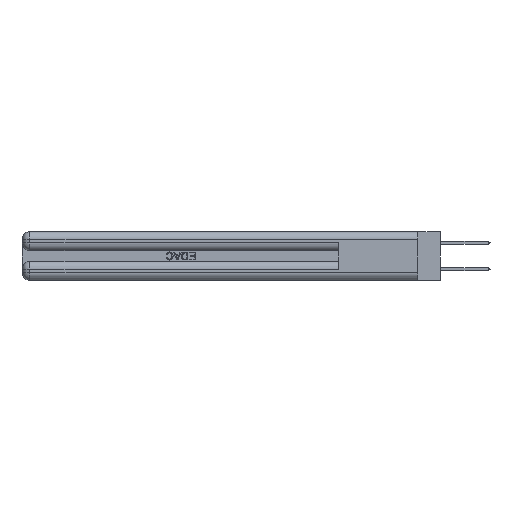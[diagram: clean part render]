
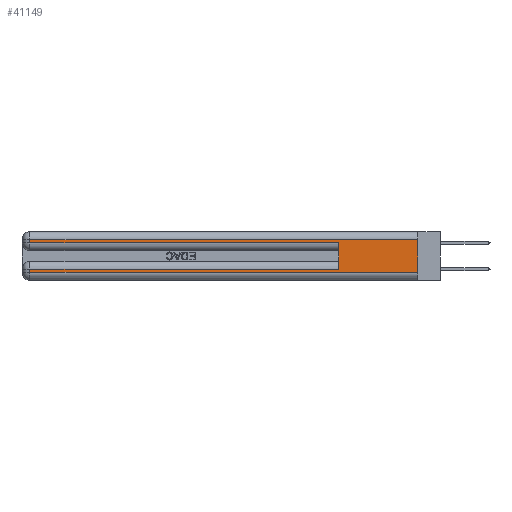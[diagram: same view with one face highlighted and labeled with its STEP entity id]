
A CAD part, left-side view. The second image highlights one B-rep face of the part: STEP entity #41149.
In plain terms, the highlighted planar face has unit normal (-1, 0, 0).
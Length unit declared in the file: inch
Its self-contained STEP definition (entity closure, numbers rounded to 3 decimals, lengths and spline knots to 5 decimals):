
#847 = CARTESIAN_POINT ( 'NONE',  ( 0., 0.6, 0.285 ) ) ;
#1053 = ORIENTED_EDGE ( 'NONE', *, *, #19100, .T. ) ;
#1753 = CARTESIAN_POINT ( 'NONE',  ( 0., 0., 0.06 ) ) ;
#2328 = LINE ( 'NONE', #5971, #9478 ) ;
#3361 = VERTEX_POINT ( 'NONE', #847 ) ;
#4598 = CARTESIAN_POINT ( 'NONE',  ( 0., 0., 0.37 ) ) ;
#5028 = VERTEX_POINT ( 'NONE', #23712 ) ;
#5296 = CARTESIAN_POINT ( 'NONE',  ( 0., 0., 0.37 ) ) ;
#5336 = EDGE_CURVE ( 'NONE', #12932, #10957, #39170, .T. ) ;
#5971 = CARTESIAN_POINT ( 'NONE',  ( 0., 0., 0.06 ) ) ;
#6801 = EDGE_CURVE ( 'NONE', #10957, #3361, #25562, .T. ) ;
#6872 = CARTESIAN_POINT ( 'NONE',  ( 0., 2.94, 0.085 ) ) ;
#7126 = ORIENTED_EDGE ( 'NONE', *, *, #5336, .T. ) ;
#7146 = VECTOR ( 'NONE', #8077, 39.37008 ) ;
#8077 = DIRECTION ( 'NONE',  ( 0., -1., 0. ) ) ;
#8470 = CARTESIAN_POINT ( 'NONE',  ( 0., 2.94, 0.285 ) ) ;
#9478 = VECTOR ( 'NONE', #9497, 39.37008 ) ;
#9497 = DIRECTION ( 'NONE',  ( 0., -1., 0. ) ) ;
#9803 = CARTESIAN_POINT ( 'NONE',  ( 0., 0., 0.085 ) ) ;
#10957 = VERTEX_POINT ( 'NONE', #8470 ) ;
#11416 = CARTESIAN_POINT ( 'NONE',  ( 0., 0., 0.285 ) ) ;
#11647 = VECTOR ( 'NONE', #25350, 39.37008 ) ;
#11980 = VERTEX_POINT ( 'NONE', #13518 ) ;
#12282 = VECTOR ( 'NONE', #25391, 39.37008 ) ;
#12932 = VERTEX_POINT ( 'NONE', #16502 ) ;
#13084 = ORIENTED_EDGE ( 'NONE', *, *, #43287, .F. ) ;
#13295 = DIRECTION ( 'NONE',  ( 0., 1., 0. ) ) ;
#13518 = CARTESIAN_POINT ( 'NONE',  ( 0., 2.94, 0.06 ) ) ;
#15785 = DIRECTION ( 'NONE',  ( 0., 0., -1. ) ) ;
#16337 = ORIENTED_EDGE ( 'NONE', *, *, #6801, .T. ) ;
#16502 = CARTESIAN_POINT ( 'NONE',  ( 0., 2.94, 0.31 ) ) ;
#16762 = EDGE_CURVE ( 'NONE', #18820, #33430, #39166, .T. ) ;
#17178 = DIRECTION ( 'NONE',  ( 0., 0., 1. ) ) ;
#17978 = ORIENTED_EDGE ( 'NONE', *, *, #25592, .F. ) ;
#18076 = LINE ( 'NONE', #38897, #44460 ) ;
#18519 = ORIENTED_EDGE ( 'NONE', *, *, #16762, .T. ) ;
#18820 = VERTEX_POINT ( 'NONE', #43369 ) ;
#19100 = EDGE_CURVE ( 'NONE', #33430, #11980, #21241, .T. ) ;
#19742 = VECTOR ( 'NONE', #13295, 39.37008 ) ;
#20513 = CARTESIAN_POINT ( 'NONE',  ( 0., 0.6, 0.145 ) ) ;
#21241 = LINE ( 'NONE', #41396, #38496 ) ;
#23015 = EDGE_CURVE ( 'NONE', #11980, #39337, #2328, .T. ) ;
#23712 = CARTESIAN_POINT ( 'NONE',  ( 0., 0., 0.31 ) ) ;
#24948 = VECTOR ( 'NONE', #17178, 39.37008 ) ;
#25350 = DIRECTION ( 'NONE',  ( 0., 0., -1. ) ) ;
#25391 = DIRECTION ( 'NONE',  ( 0., 0., -1. ) ) ;
#25562 = LINE ( 'NONE', #11416, #7146 ) ;
#25592 = EDGE_CURVE ( 'NONE', #18820, #3361, #34182, .T. ) ;
#26546 = FACE_OUTER_BOUND ( 'NONE', #34607, .T. ) ;
#30047 = AXIS2_PLACEMENT_3D ( 'NONE', #5296, #36476, #15785 ) ;
#31487 = EDGE_CURVE ( 'NONE', #5028, #12932, #18076, .T. ) ;
#33062 = PLANE ( 'NONE',  #30047 ) ;
#33430 = VERTEX_POINT ( 'NONE', #6872 ) ;
#34182 = LINE ( 'NONE', #20513, #24948 ) ;
#34607 = EDGE_LOOP ( 'NONE', ( #13084, #40602, #7126, #16337, #17978, #18519, #1053, #39027 ) ) ;
#36476 = DIRECTION ( 'NONE',  ( 1., 0., 0. ) ) ;
#38140 = DIRECTION ( 'NONE',  ( 0., 0., -1. ) ) ;
#38496 = VECTOR ( 'NONE', #38140, 39.37008 ) ;
#38897 = CARTESIAN_POINT ( 'NONE',  ( 0., 0., 0.31 ) ) ;
#39027 = ORIENTED_EDGE ( 'NONE', *, *, #23015, .T. ) ;
#39166 = LINE ( 'NONE', #9803, #19742 ) ;
#39170 = LINE ( 'NONE', #42474, #11647 ) ;
#39337 = VERTEX_POINT ( 'NONE', #1753 ) ;
#40602 = ORIENTED_EDGE ( 'NONE', *, *, #31487, .T. ) ;
#41149 = ADVANCED_FACE ( 'NONE', ( #26546 ), #33062, .F. ) ;
#41396 = CARTESIAN_POINT ( 'NONE',  ( 0., 2.94, 0.37 ) ) ;
#41931 = LINE ( 'NONE', #4598, #12282 ) ;
#42306 = DIRECTION ( 'NONE',  ( 0., 1., 0. ) ) ;
#42474 = CARTESIAN_POINT ( 'NONE',  ( 0., 2.94, 0.37 ) ) ;
#43287 = EDGE_CURVE ( 'NONE', #5028, #39337, #41931, .T. ) ;
#43369 = CARTESIAN_POINT ( 'NONE',  ( 0., 0.6, 0.085 ) ) ;
#44460 = VECTOR ( 'NONE', #42306, 39.37008 ) ;
